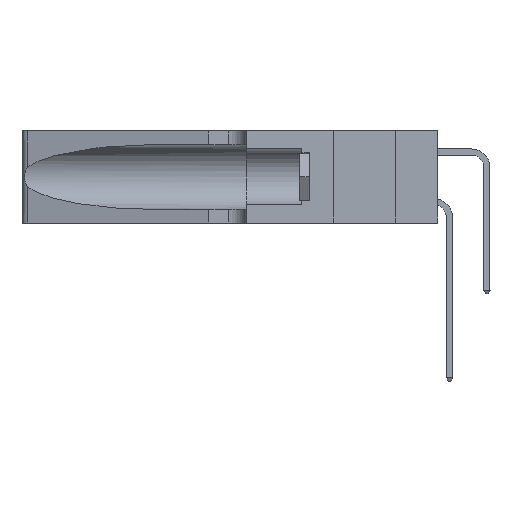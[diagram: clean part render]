
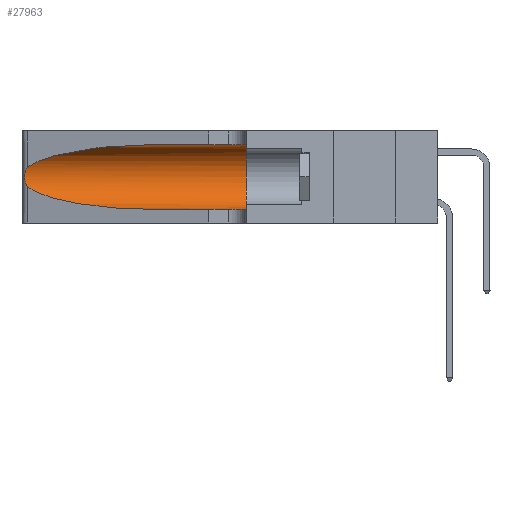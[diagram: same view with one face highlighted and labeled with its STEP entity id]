
A CAD part, left-side view. The second image highlights one B-rep face of the part: STEP entity #27963.
In plain terms, the highlighted cylindrical face has radius 3.308 mm (diameter 6.617 mm), a partial arc.
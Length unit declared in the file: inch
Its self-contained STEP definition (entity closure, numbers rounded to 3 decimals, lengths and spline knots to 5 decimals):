
#224 = EDGE_CURVE ( 'NONE', #34059, #3858, #4405, .T. ) ;
#270 = CARTESIAN_POINT ( 'NONE',  ( 0.2373, 1.15595, 0.28018 ) ) ;
#457 = EDGE_CURVE ( 'NONE', #36798, #18147, #35236, .T. ) ;
#752 = EDGE_CURVE ( 'NONE', #18147, #3858, #17553, .T. ) ;
#945 = CARTESIAN_POINT ( 'NONE',  ( 0.25487, 1.22718, 0.22369 ) ) ;
#1552 = DIRECTION ( 'NONE',  ( 0., -1., 0. ) ) ;
#2310 = CARTESIAN_POINT ( 'NONE',  ( 0.25487, 1.22718, 0.22369 ) ) ;
#3858 = VERTEX_POINT ( 'NONE', #8649 ) ;
#4405 = LINE ( 'NONE', #10224, #33908 ) ;
#5298 = CARTESIAN_POINT ( 'NONE',  ( 0.25854, 1.2359, 0.20912 ) ) ;
#5732 = EDGE_CURVE ( 'NONE', #11565, #36364, #34118, .T. ) ;
#5956 = CARTESIAN_POINT ( 'NONE',  ( 0.1305, 0.72297, 0.05475 ) ) ;
#6963 = CARTESIAN_POINT ( 'NONE',  ( 0.18966, 0.96281, 0.05475 ) ) ;
#7182 = CYLINDRICAL_SURFACE ( 'NONE', #32932, 0.13025 ) ;
#7757 = ORIENTED_EDGE ( 'NONE', *, *, #457, .F. ) ;
#8214 = ORIENTED_EDGE ( 'NONE', *, *, #37491, .T. ) ;
#8253 = CARTESIAN_POINT ( 'NONE',  ( 0.26075, 1.23896, 0.19203 ) ) ;
#8442 =( BOUNDED_CURVE ( )  B_SPLINE_CURVE ( 3, ( #12060, #26448, #270, #20778 ),
 .UNSPECIFIED., .F., .F. ) 
 B_SPLINE_CURVE_WITH_KNOTS ( ( 4, 4 ),
 ( 1.5708, 2.84003 ),
 .UNSPECIFIED. ) 
 CURVE ( )  GEOMETRIC_REPRESENTATION_ITEM ( )  RATIONAL_B_SPLINE_CURVE ( ( 1., 0.87, 0.87, 1. ) ) 
 REPRESENTATION_ITEM ( '' )  );
#8649 = CARTESIAN_POINT ( 'NONE',  ( 0.1305, 0.35, 0.05475 ) ) ;
#10224 = CARTESIAN_POINT ( 'NONE',  ( 0.1305, 1.61858, 0.05475 ) ) ;
#11185 = DIRECTION ( 'NONE',  ( 0., 1., 0. ) ) ;
#11213 = CARTESIAN_POINT ( 'NONE',  ( 0.26017, 1.23833, 0.17102 ) ) ;
#11565 = VERTEX_POINT ( 'NONE', #945 ) ;
#12060 = CARTESIAN_POINT ( 'NONE',  ( 0.1305, 0.72297, 0.31525 ) ) ;
#12751 = CARTESIAN_POINT ( 'NONE',  ( 0.2373, 1.15595, 0.08982 ) ) ;
#14150 = CARTESIAN_POINT ( 'NONE',  ( 0.25789, 1.23486, 0.15765 ) ) ;
#14702 = DIRECTION ( 'NONE',  ( 0., 0., -1. ) ) ;
#15357 = CARTESIAN_POINT ( 'NONE',  ( 0.1305, 0.35, 0.31525 ) ) ;
#15644 = DIRECTION ( 'NONE',  ( 0., -1., 0. ) ) ;
#16934 = CARTESIAN_POINT ( 'NONE',  ( 0.25639, 1.23184, 0.21858 ) ) ;
#17062 = CARTESIAN_POINT ( 'NONE',  ( 0.25555, 1.22993, 0.14849 ) ) ;
#17472 = DIRECTION ( 'NONE',  ( 0., -1., 0. ) ) ;
#17553 = CIRCLE ( 'NONE', #27271, 0.13025 ) ;
#17805 = ORIENTED_EDGE ( 'NONE', *, *, #5732, .T. ) ;
#18147 = VERTEX_POINT ( 'NONE', #15357 ) ;
#18410 = CARTESIAN_POINT ( 'NONE',  ( 0.1305, 1.61858, 0.31525 ) ) ;
#18563 = CARTESIAN_POINT ( 'NONE',  ( 0.25487, 1.22718, 0.14631 ) ) ;
#18945 = EDGE_CURVE ( 'NONE', #36364, #34059, #20773, .T. ) ;
#19826 = CARTESIAN_POINT ( 'NONE',  ( 0.25555, 1.22994, 0.2215 ) ) ;
#20773 =( BOUNDED_CURVE ( )  B_SPLINE_CURVE ( 3, ( #18563, #12751, #6963, #27264 ),
 .UNSPECIFIED., .F., .F. ) 
 B_SPLINE_CURVE_WITH_KNOTS ( ( 4, 4 ),
 ( 3.44316, 4.71239 ),
 .UNSPECIFIED. ) 
 CURVE ( )  GEOMETRIC_REPRESENTATION_ITEM ( )  RATIONAL_B_SPLINE_CURVE ( ( 1., 0.87, 0.87, 1. ) ) 
 REPRESENTATION_ITEM ( '' )  );
#20778 = CARTESIAN_POINT ( 'NONE',  ( 0.25487, 1.22718, 0.22369 ) ) ;
#22646 = FACE_OUTER_BOUND ( 'NONE', #35700, .T. ) ;
#22727 = CARTESIAN_POINT ( 'NONE',  ( 0.25787, 1.23484, 0.2124 ) ) ;
#24309 = CARTESIAN_POINT ( 'NONE',  ( 0.1305, 0.72297, 0.31525 ) ) ;
#25622 = CARTESIAN_POINT ( 'NONE',  ( 0.26018, 1.23835, 0.19895 ) ) ;
#26448 = CARTESIAN_POINT ( 'NONE',  ( 0.18966, 0.96281, 0.31525 ) ) ;
#27264 = CARTESIAN_POINT ( 'NONE',  ( 0.1305, 0.72297, 0.05475 ) ) ;
#27271 = AXIS2_PLACEMENT_3D ( 'NONE', #28461, #11185, #31329 ) ;
#27963 = ADVANCED_FACE ( 'NONE', ( #22646 ), #7182, .F. ) ;
#27984 = CARTESIAN_POINT ( 'NONE',  ( 0.25487, 1.22718, 0.14631 ) ) ;
#28160 = ORIENTED_EDGE ( 'NONE', *, *, #224, .T. ) ;
#28461 = CARTESIAN_POINT ( 'NONE',  ( 0.1305, 0.35, 0.185 ) ) ;
#28502 = CARTESIAN_POINT ( 'NONE',  ( 0.26075, 1.23896, 0.178 ) ) ;
#31329 = DIRECTION ( 'NONE',  ( 0., 0., 1. ) ) ;
#31364 = CARTESIAN_POINT ( 'NONE',  ( 0.25856, 1.23593, 0.16098 ) ) ;
#31907 = CARTESIAN_POINT ( 'NONE',  ( 0.1305, 1.61858, 0.185 ) ) ;
#32932 = AXIS2_PLACEMENT_3D ( 'NONE', #31907, #17472, #14702 ) ;
#33908 = VECTOR ( 'NONE', #1552, 39.37008 ) ;
#34059 = VERTEX_POINT ( 'NONE', #5956 ) ;
#34118 = B_SPLINE_CURVE_WITH_KNOTS ( 'NONE', 3,
 ( #2310, #19826, #16934, #22727, #5298, #25622, #8253, #28502, #11213, #31364, #14150, #34252, #17062, #37124 ),
 .UNSPECIFIED., .F., .F.,
 ( 4, 2, 2, 2, 2, 2, 4 ),
 ( 0., 0.00027, 0.00053, 0.00107, 0.0016, 0.00187, 0.00214 ),
 .UNSPECIFIED. ) ;
#34252 = CARTESIAN_POINT ( 'NONE',  ( 0.25639, 1.23186, 0.15144 ) ) ;
#34868 = ORIENTED_EDGE ( 'NONE', *, *, #18945, .T. ) ;
#35236 = LINE ( 'NONE', #18410, #36128 ) ;
#35700 = EDGE_LOOP ( 'NONE', ( #8214, #17805, #34868, #28160, #37535, #7757 ) ) ;
#36128 = VECTOR ( 'NONE', #15644, 39.37008 ) ;
#36364 = VERTEX_POINT ( 'NONE', #27984 ) ;
#36798 = VERTEX_POINT ( 'NONE', #24309 ) ;
#37124 = CARTESIAN_POINT ( 'NONE',  ( 0.25487, 1.22718, 0.14631 ) ) ;
#37491 = EDGE_CURVE ( 'NONE', #36798, #11565, #8442, .T. ) ;
#37535 = ORIENTED_EDGE ( 'NONE', *, *, #752, .F. ) ;
